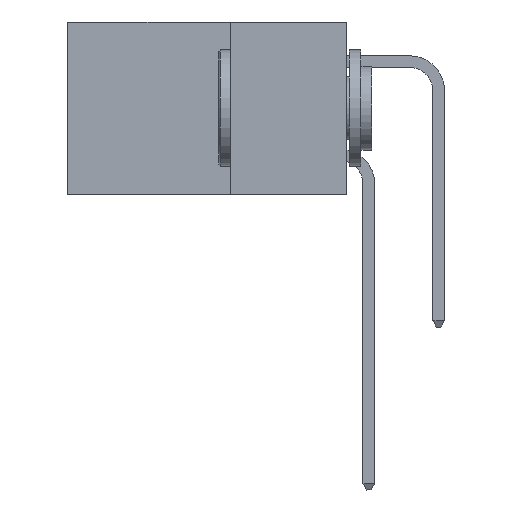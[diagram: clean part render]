
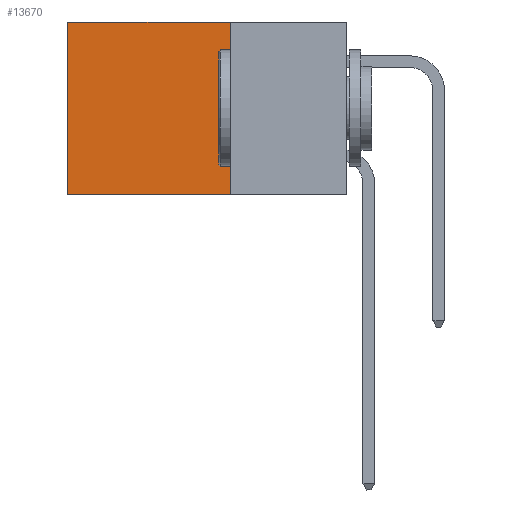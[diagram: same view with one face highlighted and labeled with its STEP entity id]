
A CAD part, left-side view. The second image highlights one B-rep face of the part: STEP entity #13670.
In plain terms, the highlighted planar face has unit normal (-1, 0, 0).
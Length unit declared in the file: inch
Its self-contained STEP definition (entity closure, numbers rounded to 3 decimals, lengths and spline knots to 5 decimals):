
#575 = CARTESIAN_POINT ( 'NONE',  ( 0.2875, 0.25, -0.37 ) ) ;
#617 = DIRECTION ( 'NONE',  ( 0., 1., 0. ) ) ;
#724 = ORIENTED_EDGE ( 'NONE', *, *, #8947, .T. ) ;
#1313 = CARTESIAN_POINT ( 'NONE',  ( 0.2875, 0.6, 0. ) ) ;
#2354 = CARTESIAN_POINT ( 'NONE',  ( 0.2875, 0.25, 0. ) ) ;
#2504 = EDGE_CURVE ( 'NONE', #7052, #16349, #6686, .T. ) ;
#2898 = CARTESIAN_POINT ( 'NONE',  ( 0.2875, 0.25, 0. ) ) ;
#2939 = LINE ( 'NONE', #1313, #17025 ) ;
#2966 = AXIS2_PLACEMENT_3D ( 'NONE', #13515, #14906, #6540 ) ;
#4357 = DIRECTION ( 'NONE',  ( 0., 0., -1. ) ) ;
#4555 = LINE ( 'NONE', #2898, #12110 ) ;
#4688 = FACE_OUTER_BOUND ( 'NONE', #12734, .T. ) ;
#5522 = VECTOR ( 'NONE', #12568, 39.37008 ) ;
#6234 = VERTEX_POINT ( 'NONE', #14984 ) ;
#6398 = EDGE_CURVE ( 'NONE', #17368, #6234, #16649, .T. ) ;
#6488 = ORIENTED_EDGE ( 'NONE', *, *, #17002, .F. ) ;
#6540 = DIRECTION ( 'NONE',  ( 0., 0., -1. ) ) ;
#6686 = LINE ( 'NONE', #575, #10899 ) ;
#7052 = VERTEX_POINT ( 'NONE', #7074 ) ;
#7074 = CARTESIAN_POINT ( 'NONE',  ( 0.2875, 0.25, -0.37 ) ) ;
#8947 = EDGE_CURVE ( 'NONE', #6234, #16349, #2939, .T. ) ;
#10124 = CARTESIAN_POINT ( 'NONE',  ( 0.2875, 0.6, -0.37 ) ) ;
#10899 = VECTOR ( 'NONE', #617, 39.37008 ) ;
#11204 = CARTESIAN_POINT ( 'NONE',  ( 0.2875, 0.25, 0. ) ) ;
#12110 = VECTOR ( 'NONE', #4357, 39.37008 ) ;
#12127 = PLANE ( 'NONE',  #2966 ) ;
#12345 = ORIENTED_EDGE ( 'NONE', *, *, #6398, .T. ) ;
#12568 = DIRECTION ( 'NONE',  ( 0., 1., 0. ) ) ;
#12734 = EDGE_LOOP ( 'NONE', ( #724, #14844, #6488, #12345 ) ) ;
#13515 = CARTESIAN_POINT ( 'NONE',  ( 0.2875, 0.25, 0. ) ) ;
#13670 = ADVANCED_FACE ( 'NONE', ( #4688 ), #12127, .F. ) ;
#14133 = DIRECTION ( 'NONE',  ( 0., 0., -1. ) ) ;
#14844 = ORIENTED_EDGE ( 'NONE', *, *, #2504, .F. ) ;
#14906 = DIRECTION ( 'NONE',  ( 1., 0., 0. ) ) ;
#14984 = CARTESIAN_POINT ( 'NONE',  ( 0.2875, 0.6, 0. ) ) ;
#16349 = VERTEX_POINT ( 'NONE', #10124 ) ;
#16649 = LINE ( 'NONE', #11204, #5522 ) ;
#17002 = EDGE_CURVE ( 'NONE', #17368, #7052, #4555, .T. ) ;
#17025 = VECTOR ( 'NONE', #14133, 39.37008 ) ;
#17368 = VERTEX_POINT ( 'NONE', #2354 ) ;
